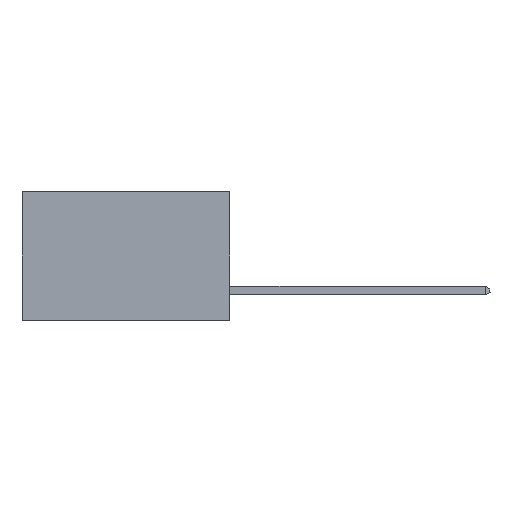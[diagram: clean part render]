
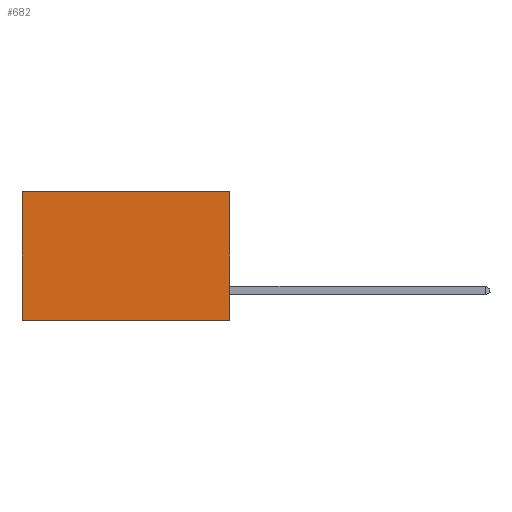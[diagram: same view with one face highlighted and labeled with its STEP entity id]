
A CAD part, left-side view. The second image highlights one B-rep face of the part: STEP entity #682.
In plain terms, the highlighted planar face has unit normal (-1, 0, 0).
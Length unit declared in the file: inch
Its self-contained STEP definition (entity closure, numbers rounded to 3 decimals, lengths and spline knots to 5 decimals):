
#1 = VECTOR ( 'NONE', #3265, 39.37008 ) ;
#51 = DIRECTION ( 'NONE',  ( 1., 0., 0. ) ) ;
#682 = ADVANCED_FACE ( 'NONE', ( #1695 ), #7919, .F. ) ;
#790 = ORIENTED_EDGE ( 'NONE', *, *, #12376, .T. ) ;
#1695 = FACE_OUTER_BOUND ( 'NONE', #14624, .T. ) ;
#3265 = DIRECTION ( 'NONE',  ( 0., 1., 0. ) ) ;
#3989 = CARTESIAN_POINT ( 'NONE',  ( 0.298, 0.6, 0. ) ) ;
#4305 = VERTEX_POINT ( 'NONE', #14128 ) ;
#5118 = EDGE_CURVE ( 'NONE', #9429, #14975, #10460, .T. ) ;
#6659 = EDGE_CURVE ( 'NONE', #4305, #9429, #7347, .T. ) ;
#7347 = LINE ( 'NONE', #13506, #10370 ) ;
#7919 = PLANE ( 'NONE',  #11995 ) ;
#8118 = DIRECTION ( 'NONE',  ( 0., 0., -1. ) ) ;
#9429 = VERTEX_POINT ( 'NONE', #12170 ) ;
#9746 = CARTESIAN_POINT ( 'NONE',  ( 0.298, 0., 0. ) ) ;
#10370 = VECTOR ( 'NONE', #11735, 39.37008 ) ;
#10460 = LINE ( 'NONE', #17037, #17030 ) ;
#10661 = ORIENTED_EDGE ( 'NONE', *, *, #6659, .F. ) ;
#10931 = CARTESIAN_POINT ( 'NONE',  ( 0.298, 0.6, 0. ) ) ;
#10959 = EDGE_CURVE ( 'NONE', #4305, #16986, #18204, .T. ) ;
#11363 = ORIENTED_EDGE ( 'NONE', *, *, #10959, .T. ) ;
#11735 = DIRECTION ( 'NONE',  ( 0., 0., -1. ) ) ;
#11995 = AXIS2_PLACEMENT_3D ( 'NONE', #9746, #51, #8118 ) ;
#12170 = CARTESIAN_POINT ( 'NONE',  ( 0.298, 0., -0.37 ) ) ;
#12376 = EDGE_CURVE ( 'NONE', #16986, #14975, #14558, .T. ) ;
#12979 = CARTESIAN_POINT ( 'NONE',  ( 0.298, 0., 0. ) ) ;
#13323 = ORIENTED_EDGE ( 'NONE', *, *, #5118, .F. ) ;
#13506 = CARTESIAN_POINT ( 'NONE',  ( 0.298, 0., 0. ) ) ;
#14128 = CARTESIAN_POINT ( 'NONE',  ( 0.298, 0., 0. ) ) ;
#14558 = LINE ( 'NONE', #3989, #18387 ) ;
#14624 = EDGE_LOOP ( 'NONE', ( #790, #13323, #10661, #11363 ) ) ;
#14975 = VERTEX_POINT ( 'NONE', #20575 ) ;
#15315 = DIRECTION ( 'NONE',  ( 0., 0., -1. ) ) ;
#16986 = VERTEX_POINT ( 'NONE', #10931 ) ;
#17030 = VECTOR ( 'NONE', #18754, 39.37008 ) ;
#17037 = CARTESIAN_POINT ( 'NONE',  ( 0.298, 0., -0.37 ) ) ;
#18204 = LINE ( 'NONE', #12979, #1 ) ;
#18387 = VECTOR ( 'NONE', #15315, 39.37008 ) ;
#18754 = DIRECTION ( 'NONE',  ( 0., 1., 0. ) ) ;
#20575 = CARTESIAN_POINT ( 'NONE',  ( 0.298, 0.6, -0.37 ) ) ;
